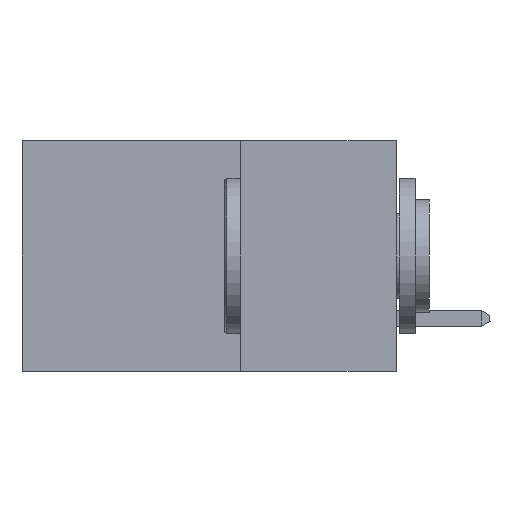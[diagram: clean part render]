
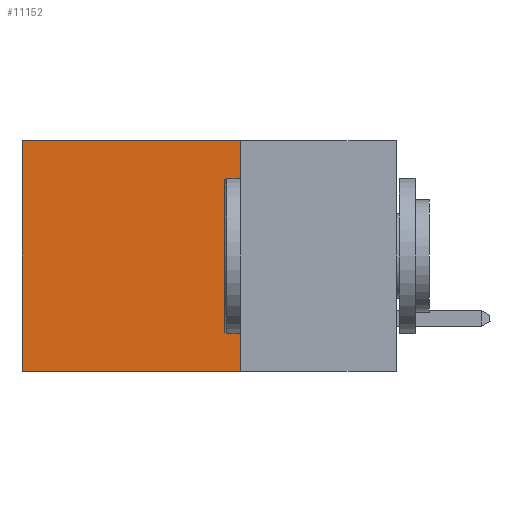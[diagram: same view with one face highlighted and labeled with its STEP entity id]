
A CAD part, left-side view. The second image highlights one B-rep face of the part: STEP entity #11152.
In plain terms, the highlighted planar face has unit normal (-1, 0, 0).
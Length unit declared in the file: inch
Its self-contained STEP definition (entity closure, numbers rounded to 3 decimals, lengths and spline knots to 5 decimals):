
#441 = LINE ( 'NONE', #1208, #15828 ) ;
#847 = VERTEX_POINT ( 'NONE', #9506 ) ;
#964 = CARTESIAN_POINT ( 'NONE',  ( 0.298, 0.6, 0. ) ) ;
#1180 = DIRECTION ( 'NONE',  ( 0., 0., -1. ) ) ;
#1199 = EDGE_CURVE ( 'NONE', #10562, #10406, #9088, .T. ) ;
#1208 = CARTESIAN_POINT ( 'NONE',  ( 0.298, 0.25, 0. ) ) ;
#1304 = DIRECTION ( 'NONE',  ( 1., 0., 0. ) ) ;
#1465 = DIRECTION ( 'NONE',  ( 0., 1., 0. ) ) ;
#1524 = VECTOR ( 'NONE', #1465, 39.37008 ) ;
#2110 = ORIENTED_EDGE ( 'NONE', *, *, #11056, .F. ) ;
#2365 = DIRECTION ( 'NONE',  ( 0., 0., -1. ) ) ;
#2966 = EDGE_CURVE ( 'NONE', #5734, #10406, #15134, .T. ) ;
#3049 = AXIS2_PLACEMENT_3D ( 'NONE', #9913, #1304, #7533 ) ;
#4068 = VECTOR ( 'NONE', #1180, 39.37008 ) ;
#4557 = ORIENTED_EDGE ( 'NONE', *, *, #1199, .T. ) ;
#5481 = ORIENTED_EDGE ( 'NONE', *, *, #2966, .F. ) ;
#5734 = VERTEX_POINT ( 'NONE', #9963 ) ;
#6472 = EDGE_CURVE ( 'NONE', #847, #10562, #11323, .T. ) ;
#7533 = DIRECTION ( 'NONE',  ( 0., 0., -1. ) ) ;
#8346 = CARTESIAN_POINT ( 'NONE',  ( 0.298, 0.6, -0.37 ) ) ;
#8351 = ORIENTED_EDGE ( 'NONE', *, *, #6472, .T. ) ;
#9088 = LINE ( 'NONE', #14758, #4068 ) ;
#9468 = FACE_OUTER_BOUND ( 'NONE', #15523, .T. ) ;
#9506 = CARTESIAN_POINT ( 'NONE',  ( 0.298, 0.25, 0. ) ) ;
#9913 = CARTESIAN_POINT ( 'NONE',  ( 0.298, 0.25, 0. ) ) ;
#9963 = CARTESIAN_POINT ( 'NONE',  ( 0.298, 0.25, -0.37 ) ) ;
#10406 = VERTEX_POINT ( 'NONE', #8346 ) ;
#10562 = VERTEX_POINT ( 'NONE', #964 ) ;
#11056 = EDGE_CURVE ( 'NONE', #847, #5734, #441, .T. ) ;
#11152 = ADVANCED_FACE ( 'NONE', ( #9468 ), #13525, .F. ) ;
#11323 = LINE ( 'NONE', #14933, #1524 ) ;
#13180 = CARTESIAN_POINT ( 'NONE',  ( 0.298, 0.25, -0.37 ) ) ;
#13233 = DIRECTION ( 'NONE',  ( 0., 1., 0. ) ) ;
#13525 = PLANE ( 'NONE',  #3049 ) ;
#13945 = VECTOR ( 'NONE', #13233, 39.37008 ) ;
#14758 = CARTESIAN_POINT ( 'NONE',  ( 0.298, 0.6, 0. ) ) ;
#14933 = CARTESIAN_POINT ( 'NONE',  ( 0.298, 0.25, 0. ) ) ;
#15134 = LINE ( 'NONE', #13180, #13945 ) ;
#15523 = EDGE_LOOP ( 'NONE', ( #4557, #5481, #2110, #8351 ) ) ;
#15828 = VECTOR ( 'NONE', #2365, 39.37008 ) ;
